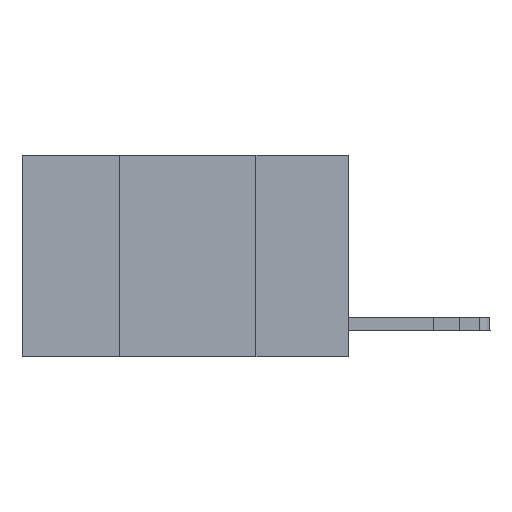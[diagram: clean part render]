
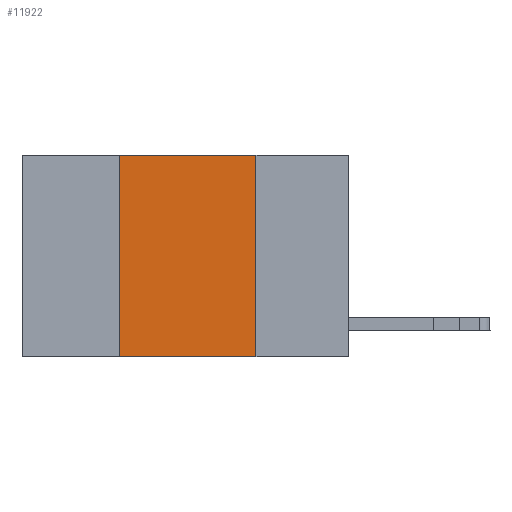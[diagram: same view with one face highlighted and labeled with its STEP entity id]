
A CAD part, left-side view. The second image highlights one B-rep face of the part: STEP entity #11922.
In plain terms, the highlighted planar face has unit normal (-1, 0, 0).
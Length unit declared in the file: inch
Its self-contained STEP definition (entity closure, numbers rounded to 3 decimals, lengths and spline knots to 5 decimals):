
#798 = ORIENTED_EDGE ( 'NONE', *, *, #4253, .T. ) ;
#1747 = LINE ( 'NONE', #22666, #3608 ) ;
#2412 = PLANE ( 'NONE',  #11221 ) ;
#3517 = VECTOR ( 'NONE', #18270, 39.37008 ) ;
#3608 = VECTOR ( 'NONE', #16850, 39.37008 ) ;
#3920 = FACE_OUTER_BOUND ( 'NONE', #19619, .T. ) ;
#4253 = EDGE_CURVE ( 'NONE', #4858, #11973, #1747, .T. ) ;
#4858 = VERTEX_POINT ( 'NONE', #10067 ) ;
#5360 = CARTESIAN_POINT ( 'NONE',  ( 0., 0.6, 0. ) ) ;
#6662 = CARTESIAN_POINT ( 'NONE',  ( 0., 0.17, 0. ) ) ;
#7095 = DIRECTION ( 'NONE',  ( 0., 0., 1. ) ) ;
#7930 = DIRECTION ( 'NONE',  ( 0., 0., -1. ) ) ;
#8934 = LINE ( 'NONE', #20184, #24124 ) ;
#9422 = EDGE_CURVE ( 'NONE', #4858, #11607, #8934, .T. ) ;
#10067 = CARTESIAN_POINT ( 'NONE',  ( 0., 0.42, -0.37 ) ) ;
#11221 = AXIS2_PLACEMENT_3D ( 'NONE', #17145, #17393, #7930 ) ;
#11607 = VERTEX_POINT ( 'NONE', #22122 ) ;
#11922 = ADVANCED_FACE ( 'NONE', ( #3920 ), #2412, .F. ) ;
#11973 = VERTEX_POINT ( 'NONE', #12514 ) ;
#12514 = CARTESIAN_POINT ( 'NONE',  ( 0., 0.17, -0.37 ) ) ;
#13564 = VERTEX_POINT ( 'NONE', #13753 ) ;
#13753 = CARTESIAN_POINT ( 'NONE',  ( 0., 0.17, 0. ) ) ;
#14197 = ORIENTED_EDGE ( 'NONE', *, *, #23344, .F. ) ;
#14738 = EDGE_CURVE ( 'NONE', #11607, #13564, #21683, .T. ) ;
#14846 = DIRECTION ( 'NONE',  ( 0., -1., 0. ) ) ;
#16850 = DIRECTION ( 'NONE',  ( 0., -1., 0. ) ) ;
#17145 = CARTESIAN_POINT ( 'NONE',  ( 0., 0.6, 0. ) ) ;
#17393 = DIRECTION ( 'NONE',  ( 1., 0., 0. ) ) ;
#18270 = DIRECTION ( 'NONE',  ( 0., 0., -1. ) ) ;
#19619 = EDGE_LOOP ( 'NONE', ( #14197, #20576, #23258, #798 ) ) ;
#20142 = LINE ( 'NONE', #6662, #3517 ) ;
#20184 = CARTESIAN_POINT ( 'NONE',  ( 0., 0.42, 0. ) ) ;
#20576 = ORIENTED_EDGE ( 'NONE', *, *, #14738, .F. ) ;
#21683 = LINE ( 'NONE', #5360, #23934 ) ;
#22122 = CARTESIAN_POINT ( 'NONE',  ( 0., 0.42, 0. ) ) ;
#22666 = CARTESIAN_POINT ( 'NONE',  ( 0., 0.6, -0.37 ) ) ;
#23258 = ORIENTED_EDGE ( 'NONE', *, *, #9422, .F. ) ;
#23344 = EDGE_CURVE ( 'NONE', #13564, #11973, #20142, .T. ) ;
#23934 = VECTOR ( 'NONE', #14846, 39.37008 ) ;
#24124 = VECTOR ( 'NONE', #7095, 39.37008 ) ;
